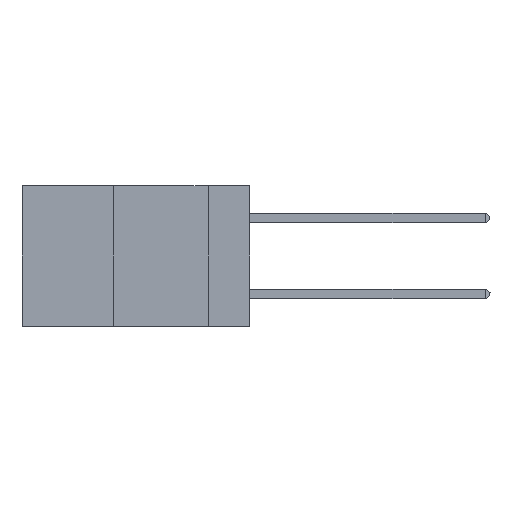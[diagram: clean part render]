
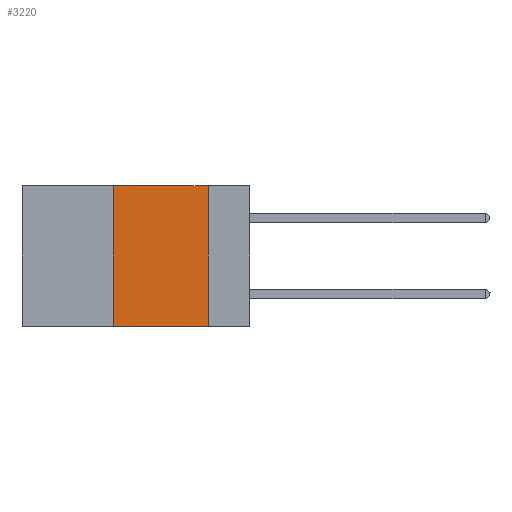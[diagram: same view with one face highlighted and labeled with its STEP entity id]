
A CAD part, left-side view. The second image highlights one B-rep face of the part: STEP entity #3220.
In plain terms, the highlighted planar face has unit normal (-1, 0, 0).
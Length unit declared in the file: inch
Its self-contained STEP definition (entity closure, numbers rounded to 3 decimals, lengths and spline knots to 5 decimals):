
#38 = EDGE_LOOP ( 'NONE', ( #15953, #9348, #4965, #4670 ) ) ;
#2097 = AXIS2_PLACEMENT_3D ( 'NONE', #12615, #17079, #3628 ) ;
#2133 = PLANE ( 'NONE',  #2097 ) ;
#3220 = ADVANCED_FACE ( 'NONE', ( #9467 ), #2133, .F. ) ;
#3440 = DIRECTION ( 'NONE',  ( 0., 0., 1. ) ) ;
#3628 = DIRECTION ( 'NONE',  ( 0., 0., -1. ) ) ;
#3807 = LINE ( 'NONE', #11353, #7760 ) ;
#4078 = EDGE_CURVE ( 'NONE', #8355, #6543, #3807, .T. ) ;
#4470 = CARTESIAN_POINT ( 'NONE',  ( 0., 0.11, 0. ) ) ;
#4491 = VECTOR ( 'NONE', #18265, 39.37008 ) ;
#4670 = ORIENTED_EDGE ( 'NONE', *, *, #10483, .T. ) ;
#4951 = LINE ( 'NONE', #5019, #4491 ) ;
#4965 = ORIENTED_EDGE ( 'NONE', *, *, #16270, .F. ) ;
#4982 = VECTOR ( 'NONE', #3440, 39.37008 ) ;
#5019 = CARTESIAN_POINT ( 'NONE',  ( 0., 0.6, 0. ) ) ;
#5764 = CARTESIAN_POINT ( 'NONE',  ( 0., 0.36, -0.37 ) ) ;
#6097 = DIRECTION ( 'NONE',  ( 0., -1., 0. ) ) ;
#6383 = LINE ( 'NONE', #16820, #4982 ) ;
#6541 = VECTOR ( 'NONE', #6097, 39.37008 ) ;
#6543 = VERTEX_POINT ( 'NONE', #8491 ) ;
#7000 = LINE ( 'NONE', #14986, #6541 ) ;
#7760 = VECTOR ( 'NONE', #14601, 39.37008 ) ;
#8325 = VERTEX_POINT ( 'NONE', #11764 ) ;
#8355 = VERTEX_POINT ( 'NONE', #4470 ) ;
#8491 = CARTESIAN_POINT ( 'NONE',  ( 0., 0.11, -0.37 ) ) ;
#9348 = ORIENTED_EDGE ( 'NONE', *, *, #9468, .F. ) ;
#9467 = FACE_OUTER_BOUND ( 'NONE', #38, .T. ) ;
#9468 = EDGE_CURVE ( 'NONE', #8325, #8355, #4951, .T. ) ;
#10483 = EDGE_CURVE ( 'NONE', #12223, #6543, #7000, .T. ) ;
#11353 = CARTESIAN_POINT ( 'NONE',  ( 0., 0.11, 0. ) ) ;
#11764 = CARTESIAN_POINT ( 'NONE',  ( 0., 0.36, 0. ) ) ;
#12223 = VERTEX_POINT ( 'NONE', #5764 ) ;
#12615 = CARTESIAN_POINT ( 'NONE',  ( 0., 0.6, 0. ) ) ;
#14601 = DIRECTION ( 'NONE',  ( 0., 0., -1. ) ) ;
#14986 = CARTESIAN_POINT ( 'NONE',  ( 0., 0.6, -0.37 ) ) ;
#15953 = ORIENTED_EDGE ( 'NONE', *, *, #4078, .F. ) ;
#16270 = EDGE_CURVE ( 'NONE', #12223, #8325, #6383, .T. ) ;
#16820 = CARTESIAN_POINT ( 'NONE',  ( 0., 0.36, 0. ) ) ;
#17079 = DIRECTION ( 'NONE',  ( 1., 0., 0. ) ) ;
#18265 = DIRECTION ( 'NONE',  ( 0., -1., 0. ) ) ;
